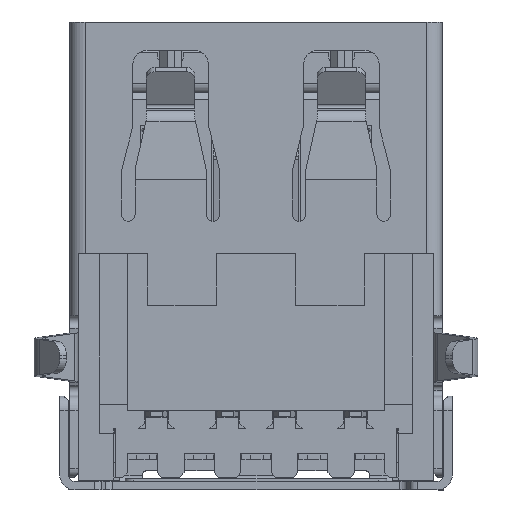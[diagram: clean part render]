
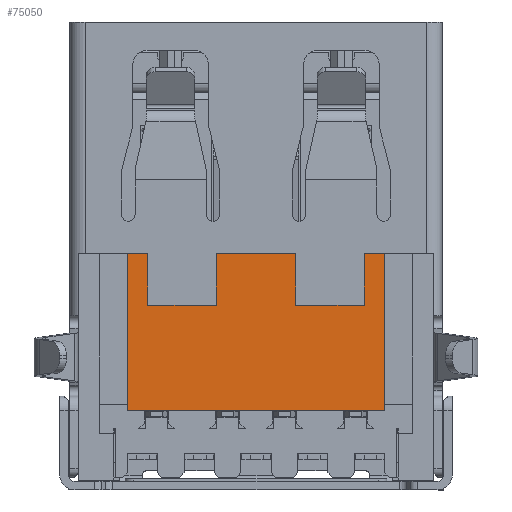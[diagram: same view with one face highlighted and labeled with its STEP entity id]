
A CAD part, front view. The second image highlights one B-rep face of the part: STEP entity #75050.
In plain terms, the highlighted face is planar.
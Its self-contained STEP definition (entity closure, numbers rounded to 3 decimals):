
#1902 = CARTESIAN_POINT ( 'NONE',  ( 0., 5.62, 4.13 ) ) ;
#2289 = VECTOR ( 'NONE', #31726, 1000. ) ;
#2727 = EDGE_CURVE ( 'NONE', #40512, #55390, #43296, .T. ) ;
#4559 = CARTESIAN_POINT ( 'NONE',  ( -6.225, -2.33, 4.13 ) ) ;
#5543 = VERTEX_POINT ( 'NONE', #25440 ) ;
#6150 = ORIENTED_EDGE ( 'NONE', *, *, #61614, .T. ) ;
#6520 = ORIENTED_EDGE ( 'NONE', *, *, #22024, .T. ) ;
#7082 = CARTESIAN_POINT ( 'NONE',  ( -1.4, -0.53, 4.13 ) ) ;
#7818 = VECTOR ( 'NONE', #28119, 1000. ) ;
#9359 = ORIENTED_EDGE ( 'NONE', *, *, #35796, .T. ) ;
#9956 = DIRECTION ( 'NONE',  ( 0., -1., 0. ) ) ;
#13516 = FACE_OUTER_BOUND ( 'NONE', #61186, .T. ) ;
#13544 = LINE ( 'NONE', #54471, #48534 ) ;
#13566 = VERTEX_POINT ( 'NONE', #16296 ) ;
#14482 = LINE ( 'NONE', #38020, #75755 ) ;
#14680 = AXIS2_PLACEMENT_3D ( 'NONE', #1902, #24320, #65666 ) ;
#14760 = LINE ( 'NONE', #68443, #39711 ) ;
#16296 = CARTESIAN_POINT ( 'NONE',  ( -3.8, -0.53, 4.13 ) ) ;
#16342 = EDGE_CURVE ( 'NONE', #44480, #50746, #23085, .T. ) ;
#16710 = EDGE_CURVE ( 'NONE', #21065, #55390, #16810, .T. ) ;
#16810 = LINE ( 'NONE', #33810, #74514 ) ;
#17301 = CARTESIAN_POINT ( 'NONE',  ( 4.5, 5.62, 4.13 ) ) ;
#18895 = CARTESIAN_POINT ( 'NONE',  ( 4.5, 3.17, 4.13 ) ) ;
#19024 = CARTESIAN_POINT ( 'NONE',  ( -4.5, -2.33, 4.13 ) ) ;
#19675 = PLANE ( 'NONE',  #14680 ) ;
#21065 = VERTEX_POINT ( 'NONE', #43202 ) ;
#22024 = EDGE_CURVE ( 'NONE', #48451, #31252, #32102, .T. ) ;
#22601 = DIRECTION ( 'NONE',  ( -1., 0., 0. ) ) ;
#23085 = LINE ( 'NONE', #4559, #7818 ) ;
#23516 = VERTEX_POINT ( 'NONE', #18895 ) ;
#23662 = ORIENTED_EDGE ( 'NONE', *, *, #47569, .T. ) ;
#24320 = DIRECTION ( 'NONE',  ( 0., 0., 1. ) ) ;
#25440 = CARTESIAN_POINT ( 'NONE',  ( 3.8, -0.53, 4.13 ) ) ;
#28119 = DIRECTION ( 'NONE',  ( -1., 0., 0. ) ) ;
#28193 = LINE ( 'NONE', #35097, #52057 ) ;
#29927 = CARTESIAN_POINT ( 'NONE',  ( 1.4, -2.33, 4.13 ) ) ;
#31252 = VERTEX_POINT ( 'NONE', #71685 ) ;
#31726 = DIRECTION ( 'NONE',  ( 0., -1., 0. ) ) ;
#32102 = LINE ( 'NONE', #37502, #2289 ) ;
#32748 = ORIENTED_EDGE ( 'NONE', *, *, #50095, .T. ) ;
#33810 = CARTESIAN_POINT ( 'NONE',  ( -6.225, -2.33, 4.13 ) ) ;
#34140 = VECTOR ( 'NONE', #9956, 1000. ) ;
#35097 = CARTESIAN_POINT ( 'NONE',  ( 0., 3.17, 4.13 ) ) ;
#35796 = EDGE_CURVE ( 'NONE', #21065, #13566, #53856, .T. ) ;
#36120 = ORIENTED_EDGE ( 'NONE', *, *, #2727, .T. ) ;
#36382 = CARTESIAN_POINT ( 'NONE',  ( 0., -2.33, 4.13 ) ) ;
#37104 = LINE ( 'NONE', #44072, #47162 ) ;
#37502 = CARTESIAN_POINT ( 'NONE',  ( -1.4, 5.62, 4.13 ) ) ;
#37623 = DIRECTION ( 'NONE',  ( 0., -1., 0. ) ) ;
#38020 = CARTESIAN_POINT ( 'NONE',  ( 3.8, 5.62, 4.13 ) ) ;
#39615 = CARTESIAN_POINT ( 'NONE',  ( 3.8, -2.33, 4.13 ) ) ;
#39711 = VECTOR ( 'NONE', #43716, 1000. ) ;
#40512 = VERTEX_POINT ( 'NONE', #55636 ) ;
#41055 = ORIENTED_EDGE ( 'NONE', *, *, #16342, .F. ) ;
#41083 = ORIENTED_EDGE ( 'NONE', *, *, #16710, .F. ) ;
#41425 = LINE ( 'NONE', #36382, #74695 ) ;
#42251 = DIRECTION ( 'NONE',  ( 0., 1., 0. ) ) ;
#43202 = CARTESIAN_POINT ( 'NONE',  ( -3.8, -2.33, 4.13 ) ) ;
#43296 = LINE ( 'NONE', #61478, #34140 ) ;
#43716 = DIRECTION ( 'NONE',  ( 1., 0., 0. ) ) ;
#44072 = CARTESIAN_POINT ( 'NONE',  ( 1.4, 5.62, 4.13 ) ) ;
#44480 = VERTEX_POINT ( 'NONE', #65675 ) ;
#44637 = VERTEX_POINT ( 'NONE', #29927 ) ;
#44718 = ORIENTED_EDGE ( 'NONE', *, *, #71347, .T. ) ;
#46548 = CARTESIAN_POINT ( 'NONE',  ( -3.8, 5.62, 4.13 ) ) ;
#46806 = VERTEX_POINT ( 'NONE', #74841 ) ;
#47162 = VECTOR ( 'NONE', #61474, 1000. ) ;
#47230 = DIRECTION ( 'NONE',  ( 1., 0., 0. ) ) ;
#47569 = EDGE_CURVE ( 'NONE', #44480, #23516, #75320, .T. ) ;
#48451 = VERTEX_POINT ( 'NONE', #7082 ) ;
#48534 = VECTOR ( 'NONE', #48676, 1000. ) ;
#48676 = DIRECTION ( 'NONE',  ( 1., 0., 0. ) ) ;
#49265 = VECTOR ( 'NONE', #42251, 1000. ) ;
#50095 = EDGE_CURVE ( 'NONE', #44637, #46806, #37104, .T. ) ;
#50263 = EDGE_CURVE ( 'NONE', #13566, #48451, #14760, .T. ) ;
#50746 = VERTEX_POINT ( 'NONE', #39615 ) ;
#52057 = VECTOR ( 'NONE', #57173, 1000. ) ;
#52838 = DIRECTION ( 'NONE',  ( 0., 1., 0. ) ) ;
#52869 = EDGE_CURVE ( 'NONE', #46806, #5543, #13544, .T. ) ;
#53856 = LINE ( 'NONE', #46548, #49265 ) ;
#54471 = CARTESIAN_POINT ( 'NONE',  ( 3.8, -0.53, 4.13 ) ) ;
#54494 = ORIENTED_EDGE ( 'NONE', *, *, #50263, .T. ) ;
#55390 = VERTEX_POINT ( 'NONE', #19024 ) ;
#55636 = CARTESIAN_POINT ( 'NONE',  ( -4.5, 3.17, 4.13 ) ) ;
#57173 = DIRECTION ( 'NONE',  ( -1., 0., 0. ) ) ;
#57575 = VECTOR ( 'NONE', #52838, 1000. ) ;
#59246 = ORIENTED_EDGE ( 'NONE', *, *, #59341, .T. ) ;
#59341 = EDGE_CURVE ( 'NONE', #23516, #40512, #28193, .T. ) ;
#61186 = EDGE_LOOP ( 'NONE', ( #36120, #41083, #9359, #54494, #6520, #44718, #32748, #70346, #6150, #41055, #23662, #59246 ) ) ;
#61474 = DIRECTION ( 'NONE',  ( 0., 1., 0. ) ) ;
#61478 = CARTESIAN_POINT ( 'NONE',  ( -4.5, 5.62, 4.13 ) ) ;
#61614 = EDGE_CURVE ( 'NONE', #5543, #50746, #14482, .T. ) ;
#65666 = DIRECTION ( 'NONE',  ( 1., 0., 0. ) ) ;
#65675 = CARTESIAN_POINT ( 'NONE',  ( 4.5, -2.33, 4.13 ) ) ;
#68443 = CARTESIAN_POINT ( 'NONE',  ( -1.4, -0.53, 4.13 ) ) ;
#70346 = ORIENTED_EDGE ( 'NONE', *, *, #52869, .T. ) ;
#71347 = EDGE_CURVE ( 'NONE', #31252, #44637, #41425, .T. ) ;
#71685 = CARTESIAN_POINT ( 'NONE',  ( -1.4, -2.33, 4.13 ) ) ;
#74514 = VECTOR ( 'NONE', #22601, 1000. ) ;
#74695 = VECTOR ( 'NONE', #47230, 1000. ) ;
#74841 = CARTESIAN_POINT ( 'NONE',  ( 1.4, -0.53, 4.13 ) ) ;
#75050 = ADVANCED_FACE ( 'NONE', ( #13516 ), #19675, .T. ) ;
#75320 = LINE ( 'NONE', #17301, #57575 ) ;
#75755 = VECTOR ( 'NONE', #37623, 1000. ) ;
